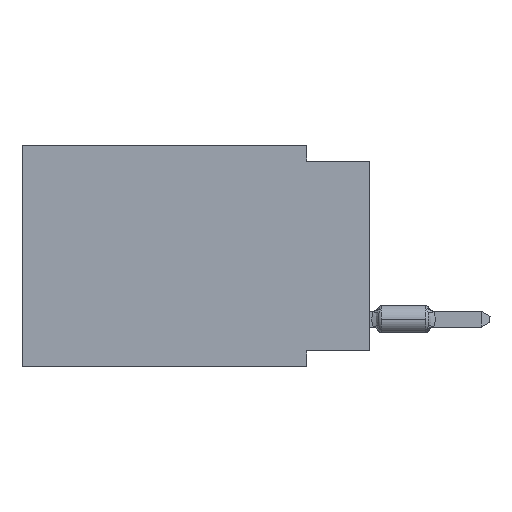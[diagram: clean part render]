
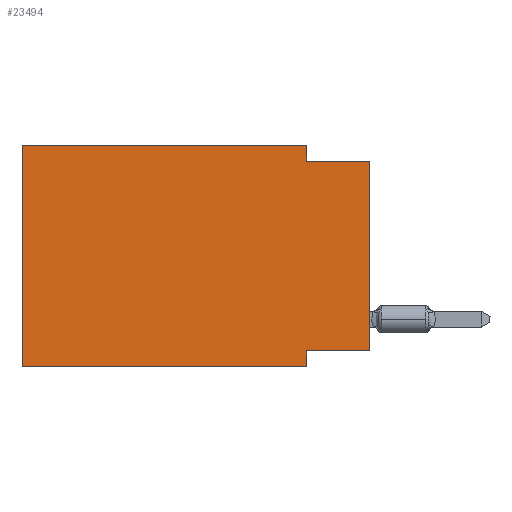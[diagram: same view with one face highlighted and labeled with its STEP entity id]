
A CAD part, left-side view. The second image highlights one B-rep face of the part: STEP entity #23494.
In plain terms, the highlighted planar face has unit normal (-1, 0, 0).
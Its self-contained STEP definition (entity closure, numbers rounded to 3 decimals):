
#984 = DIRECTION ( 'NONE',  ( 0., 0., -1. ) ) ;
#998 = EDGE_LOOP ( 'NONE', ( #67990, #3315, #30904, #41122, #36675, #24179, #32730, #37726 ) ) ;
#3214 = VERTEX_POINT ( 'NONE', #18700 ) ;
#3315 = ORIENTED_EDGE ( 'NONE', *, *, #49023, .F. ) ;
#3806 = CARTESIAN_POINT ( 'NONE',  ( 0., 0., -0.635 ) ) ;
#4251 = CARTESIAN_POINT ( 'NONE',  ( 0., 13.97, 0. ) ) ;
#4959 = CARTESIAN_POINT ( 'NONE',  ( 0., 0., -8.255 ) ) ;
#5825 = CARTESIAN_POINT ( 'NONE',  ( 0., 2.54, -8.89 ) ) ;
#8526 = CARTESIAN_POINT ( 'NONE',  ( 0., 13.97, 0. ) ) ;
#9640 = LINE ( 'NONE', #30296, #26584 ) ;
#10796 = VERTEX_POINT ( 'NONE', #5825 ) ;
#11157 = FACE_OUTER_BOUND ( 'NONE', #998, .T. ) ;
#13638 = DIRECTION ( 'NONE',  ( 0., -1., 0. ) ) ;
#14658 = VECTOR ( 'NONE', #15418, 1000. ) ;
#15418 = DIRECTION ( 'NONE',  ( 0., 0., -1. ) ) ;
#15951 = LINE ( 'NONE', #26131, #43879 ) ;
#16847 = CARTESIAN_POINT ( 'NONE',  ( 0., 2.54, -8.255 ) ) ;
#17026 = EDGE_CURVE ( 'NONE', #17246, #10796, #25814, .T. ) ;
#17246 = VERTEX_POINT ( 'NONE', #55581 ) ;
#17402 = DIRECTION ( 'NONE',  ( 0., 1., 0. ) ) ;
#18700 = CARTESIAN_POINT ( 'NONE',  ( 0., 2.54, 0. ) ) ;
#18755 = DIRECTION ( 'NONE',  ( 0., -1., 0. ) ) ;
#19997 = DIRECTION ( 'NONE',  ( 0., 0., 1. ) ) ;
#22531 = AXIS2_PLACEMENT_3D ( 'NONE', #26909, #53220, #984 ) ;
#23494 = ADVANCED_FACE ( 'NONE', ( #11157 ), #59870, .F. ) ;
#23825 = EDGE_CURVE ( 'NONE', #3214, #25199, #15951, .T. ) ;
#24179 = ORIENTED_EDGE ( 'NONE', *, *, #17026, .T. ) ;
#24569 = LINE ( 'NONE', #4251, #67202 ) ;
#25141 = LINE ( 'NONE', #58409, #39387 ) ;
#25199 = VERTEX_POINT ( 'NONE', #50218 ) ;
#25814 = LINE ( 'NONE', #59102, #55484 ) ;
#26131 = CARTESIAN_POINT ( 'NONE',  ( 0., 2.54, 0. ) ) ;
#26584 = VECTOR ( 'NONE', #18755, 1000. ) ;
#26624 = LINE ( 'NONE', #42070, #14658 ) ;
#26909 = CARTESIAN_POINT ( 'NONE',  ( 0., 13.97, 0. ) ) ;
#30296 = CARTESIAN_POINT ( 'NONE',  ( 0., 0., -0.635 ) ) ;
#30904 = ORIENTED_EDGE ( 'NONE', *, *, #23825, .F. ) ;
#31804 = VECTOR ( 'NONE', #17402, 1000. ) ;
#32058 = EDGE_CURVE ( 'NONE', #34139, #35487, #44404, .T. ) ;
#32730 = ORIENTED_EDGE ( 'NONE', *, *, #38172, .F. ) ;
#33049 = VERTEX_POINT ( 'NONE', #3806 ) ;
#34139 = VERTEX_POINT ( 'NONE', #4959 ) ;
#35487 = VERTEX_POINT ( 'NONE', #16847 ) ;
#36675 = ORIENTED_EDGE ( 'NONE', *, *, #39160, .F. ) ;
#37726 = ORIENTED_EDGE ( 'NONE', *, *, #32058, .F. ) ;
#38172 = EDGE_CURVE ( 'NONE', #35487, #10796, #26624, .T. ) ;
#39160 = EDGE_CURVE ( 'NONE', #17246, #46605, #24569, .T. ) ;
#39387 = VECTOR ( 'NONE', #68590, 1000. ) ;
#39819 = CARTESIAN_POINT ( 'NONE',  ( 0., 0., -8.255 ) ) ;
#40630 = LINE ( 'NONE', #56411, #57858 ) ;
#41122 = ORIENTED_EDGE ( 'NONE', *, *, #41652, .F. ) ;
#41652 = EDGE_CURVE ( 'NONE', #46605, #3214, #40630, .T. ) ;
#42070 = CARTESIAN_POINT ( 'NONE',  ( 0., 2.54, -8.89 ) ) ;
#43313 = DIRECTION ( 'NONE',  ( 0., 0., -1. ) ) ;
#43879 = VECTOR ( 'NONE', #43313, 1000. ) ;
#44404 = LINE ( 'NONE', #39819, #31804 ) ;
#46605 = VERTEX_POINT ( 'NONE', #8526 ) ;
#48215 = DIRECTION ( 'NONE',  ( 0., -1., 0. ) ) ;
#49023 = EDGE_CURVE ( 'NONE', #25199, #33049, #9640, .T. ) ;
#50218 = CARTESIAN_POINT ( 'NONE',  ( 0., 2.54, -0.635 ) ) ;
#53220 = DIRECTION ( 'NONE',  ( 1., 0., 0. ) ) ;
#55484 = VECTOR ( 'NONE', #48215, 1000. ) ;
#55581 = CARTESIAN_POINT ( 'NONE',  ( 0., 13.97, -8.89 ) ) ;
#56411 = CARTESIAN_POINT ( 'NONE',  ( 0., 13.97, 0. ) ) ;
#57858 = VECTOR ( 'NONE', #13638, 1000. ) ;
#58409 = CARTESIAN_POINT ( 'NONE',  ( 0., 0., 0. ) ) ;
#59102 = CARTESIAN_POINT ( 'NONE',  ( 0., 13.97, -8.89 ) ) ;
#59870 = PLANE ( 'NONE',  #22531 ) ;
#66721 = EDGE_CURVE ( 'NONE', #34139, #33049, #25141, .T. ) ;
#67202 = VECTOR ( 'NONE', #19997, 1000. ) ;
#67990 = ORIENTED_EDGE ( 'NONE', *, *, #66721, .T. ) ;
#68590 = DIRECTION ( 'NONE',  ( 0., 0., 1. ) ) ;
